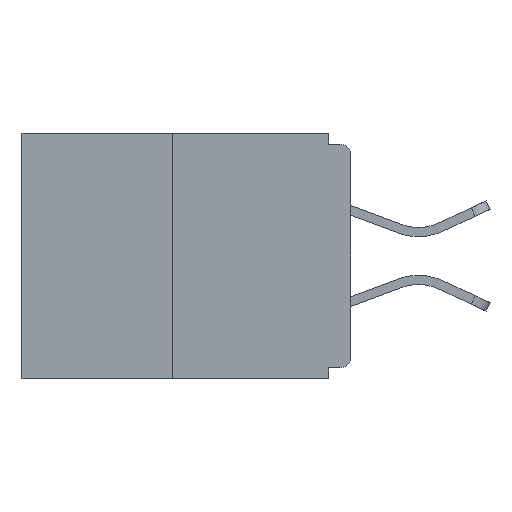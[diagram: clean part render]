
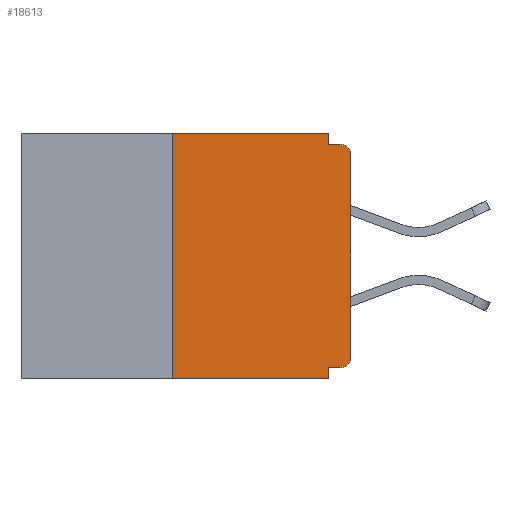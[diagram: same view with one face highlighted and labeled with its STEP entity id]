
A CAD part, left-side view. The second image highlights one B-rep face of the part: STEP entity #18613.
In plain terms, the highlighted planar face has unit normal (-1, 0, 0).
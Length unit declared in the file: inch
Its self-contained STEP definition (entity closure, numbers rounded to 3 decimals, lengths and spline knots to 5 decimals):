
#394 = VERTEX_POINT ( 'NONE', #13292 ) ;
#441 = DIRECTION ( 'NONE',  ( 0., 0., 1. ) ) ;
#704 = EDGE_CURVE ( 'NONE', #14406, #17553, #18019, .T. ) ;
#1189 = CARTESIAN_POINT ( 'NONE',  ( 0., 0.015, -0.03 ) ) ;
#1563 = VERTEX_POINT ( 'NONE', #19143 ) ;
#1718 = DIRECTION ( 'NONE',  ( 0., -1., 0. ) ) ;
#2060 = CARTESIAN_POINT ( 'NONE',  ( 0., 0., -0.015 ) ) ;
#2762 = PLANE ( 'NONE',  #15058 ) ;
#2794 = EDGE_CURVE ( 'NONE', #1563, #16474, #17006, .T. ) ;
#2988 = ORIENTED_EDGE ( 'NONE', *, *, #11015, .T. ) ;
#3069 = AXIS2_PLACEMENT_3D ( 'NONE', #1189, #22242, #24576 ) ;
#3238 = EDGE_CURVE ( 'NONE', #15497, #16496, #24684, .T. ) ;
#3583 = DIRECTION ( 'NONE',  ( 0., 0., -1. ) ) ;
#4257 = DIRECTION ( 'NONE',  ( 0., 1., 0. ) ) ;
#4357 = ORIENTED_EDGE ( 'NONE', *, *, #27560, .T. ) ;
#4609 = ORIENTED_EDGE ( 'NONE', *, *, #22556, .F. ) ;
#5186 = VECTOR ( 'NONE', #22197, 39.37008 ) ;
#5917 = DIRECTION ( 'NONE',  ( 0., -1., 0. ) ) ;
#6300 = ORIENTED_EDGE ( 'NONE', *, *, #20120, .F. ) ;
#6414 = CARTESIAN_POINT ( 'NONE',  ( 0., 0.031, -0.328 ) ) ;
#6894 = LINE ( 'NONE', #20306, #23381 ) ;
#6980 = VERTEX_POINT ( 'NONE', #19810 ) ;
#7235 = ORIENTED_EDGE ( 'NONE', *, *, #17156, .T. ) ;
#7807 = EDGE_LOOP ( 'NONE', ( #12369, #27290, #7235, #6300, #25451, #15009, #2988, #4357, #13120, #4609 ) ) ;
#8199 = VECTOR ( 'NONE', #23548, 39.37008 ) ;
#9009 = DIRECTION ( 'NONE',  ( 1., 0., 0. ) ) ;
#9674 = CARTESIAN_POINT ( 'NONE',  ( 0., 0.031, -0.343 ) ) ;
#9946 = DIRECTION ( 'NONE',  ( -1., 0., 0. ) ) ;
#11015 = EDGE_CURVE ( 'NONE', #15069, #6980, #23464, .T. ) ;
#11363 = CARTESIAN_POINT ( 'NONE',  ( 0., 0.25, 0. ) ) ;
#11381 = VECTOR ( 'NONE', #5917, 39.37008 ) ;
#12321 = VECTOR ( 'NONE', #1718, 39.37008 ) ;
#12369 = ORIENTED_EDGE ( 'NONE', *, *, #704, .F. ) ;
#12988 = EDGE_CURVE ( 'NONE', #1563, #15069, #15610, .T. ) ;
#13030 = VECTOR ( 'NONE', #441, 39.37008 ) ;
#13120 = ORIENTED_EDGE ( 'NONE', *, *, #3238, .F. ) ;
#13292 = CARTESIAN_POINT ( 'NONE',  ( 0., 0.25, -0.343 ) ) ;
#13509 = CARTESIAN_POINT ( 'NONE',  ( 0., 0.031, -0.343 ) ) ;
#13936 = DIRECTION ( 'NONE',  ( 0., 0., 1. ) ) ;
#14406 = VERTEX_POINT ( 'NONE', #11363 ) ;
#15009 = ORIENTED_EDGE ( 'NONE', *, *, #12988, .T. ) ;
#15058 = AXIS2_PLACEMENT_3D ( 'NONE', #21894, #9009, #26221 ) ;
#15069 = VERTEX_POINT ( 'NONE', #22498 ) ;
#15497 = VERTEX_POINT ( 'NONE', #16463 ) ;
#15610 = CIRCLE ( 'NONE', #23778, 0.015 ) ;
#16463 = CARTESIAN_POINT ( 'NONE',  ( 0., 0.031, -0.015 ) ) ;
#16474 = VERTEX_POINT ( 'NONE', #6414 ) ;
#16496 = VERTEX_POINT ( 'NONE', #17133 ) ;
#16745 = DIRECTION ( 'NONE',  ( 0., 0., -1. ) ) ;
#17006 = LINE ( 'NONE', #23762, #21024 ) ;
#17036 = FACE_OUTER_BOUND ( 'NONE', #7807, .T. ) ;
#17110 = LINE ( 'NONE', #25270, #11381 ) ;
#17133 = CARTESIAN_POINT ( 'NONE',  ( 0., 0.015, -0.015 ) ) ;
#17156 = EDGE_CURVE ( 'NONE', #394, #24385, #17110, .T. ) ;
#17553 = VERTEX_POINT ( 'NONE', #18102 ) ;
#18019 = LINE ( 'NONE', #23127, #12321 ) ;
#18102 = CARTESIAN_POINT ( 'NONE',  ( 0., 0.031, 0. ) ) ;
#18339 = LINE ( 'NONE', #9674, #5186 ) ;
#18613 = ADVANCED_FACE ( 'NONE', ( #17036 ), #2762, .F. ) ;
#18994 = EDGE_CURVE ( 'NONE', #394, #14406, #6894, .T. ) ;
#19143 = CARTESIAN_POINT ( 'NONE',  ( 0., 0.015, -0.328 ) ) ;
#19242 = VECTOR ( 'NONE', #16745, 39.37008 ) ;
#19810 = CARTESIAN_POINT ( 'NONE',  ( 0., 0., -0.03 ) ) ;
#20120 = EDGE_CURVE ( 'NONE', #16474, #24385, #18339, .T. ) ;
#20306 = CARTESIAN_POINT ( 'NONE',  ( 0., 0.25, 0. ) ) ;
#21024 = VECTOR ( 'NONE', #4257, 39.37008 ) ;
#21894 = CARTESIAN_POINT ( 'NONE',  ( 0., 0.46, 0. ) ) ;
#22197 = DIRECTION ( 'NONE',  ( 0., 0., -1. ) ) ;
#22242 = DIRECTION ( 'NONE',  ( -1., 0., 0. ) ) ;
#22498 = CARTESIAN_POINT ( 'NONE',  ( 0., 0., -0.313 ) ) ;
#22556 = EDGE_CURVE ( 'NONE', #17553, #15497, #22598, .T. ) ;
#22598 = LINE ( 'NONE', #23020, #19242 ) ;
#23020 = CARTESIAN_POINT ( 'NONE',  ( 0., 0.031, 0. ) ) ;
#23127 = CARTESIAN_POINT ( 'NONE',  ( 0., 0.46, 0. ) ) ;
#23381 = VECTOR ( 'NONE', #13936, 39.37008 ) ;
#23464 = LINE ( 'NONE', #24399, #13030 ) ;
#23548 = DIRECTION ( 'NONE',  ( 0., -1., 0. ) ) ;
#23762 = CARTESIAN_POINT ( 'NONE',  ( 0., 0., -0.328 ) ) ;
#23778 = AXIS2_PLACEMENT_3D ( 'NONE', #26867, #9946, #3583 ) ;
#23822 = CIRCLE ( 'NONE', #3069, 0.015 ) ;
#24385 = VERTEX_POINT ( 'NONE', #13509 ) ;
#24399 = CARTESIAN_POINT ( 'NONE',  ( 0., 0., 0. ) ) ;
#24576 = DIRECTION ( 'NONE',  ( 0., 0., -1. ) ) ;
#24684 = LINE ( 'NONE', #2060, #8199 ) ;
#25270 = CARTESIAN_POINT ( 'NONE',  ( 0., 0.46, -0.343 ) ) ;
#25451 = ORIENTED_EDGE ( 'NONE', *, *, #2794, .F. ) ;
#26221 = DIRECTION ( 'NONE',  ( 0., 0., -1. ) ) ;
#26867 = CARTESIAN_POINT ( 'NONE',  ( 0., 0.015, -0.313 ) ) ;
#27290 = ORIENTED_EDGE ( 'NONE', *, *, #18994, .F. ) ;
#27560 = EDGE_CURVE ( 'NONE', #6980, #16496, #23822, .T. ) ;
